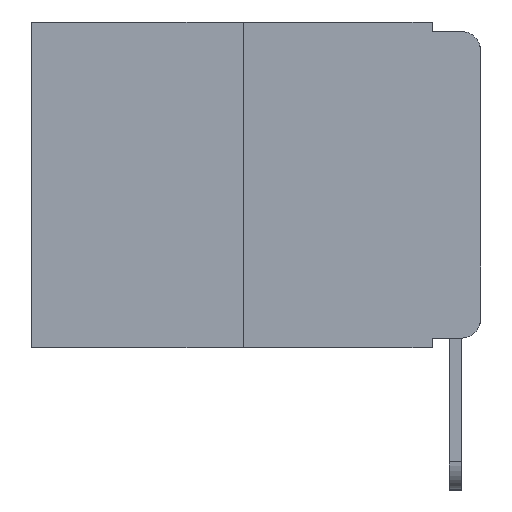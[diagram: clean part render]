
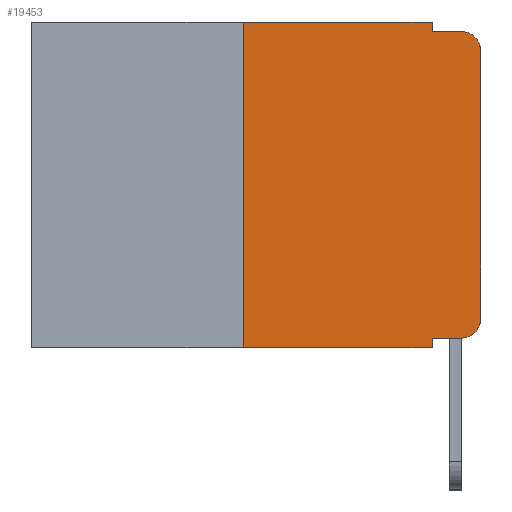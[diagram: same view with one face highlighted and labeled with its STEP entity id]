
A CAD part, left-side view. The second image highlights one B-rep face of the part: STEP entity #19453.
In plain terms, the highlighted planar face has unit normal (-1, 0, 0).
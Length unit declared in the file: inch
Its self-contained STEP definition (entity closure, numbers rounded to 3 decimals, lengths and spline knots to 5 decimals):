
#561 = CARTESIAN_POINT ( 'NONE',  ( 0., 0.02, -0.333 ) ) ;
#791 = LINE ( 'NONE', #21760, #6153 ) ;
#877 = CARTESIAN_POINT ( 'NONE',  ( 0., 0.473, 0. ) ) ;
#1076 = EDGE_CURVE ( 'NONE', #20638, #2877, #19353, .T. ) ;
#1292 = VERTEX_POINT ( 'NONE', #16886 ) ;
#1358 = LINE ( 'NONE', #10481, #18999 ) ;
#1456 = ORIENTED_EDGE ( 'NONE', *, *, #20039, .T. ) ;
#1734 = ORIENTED_EDGE ( 'NONE', *, *, #22478, .F. ) ;
#2273 = VERTEX_POINT ( 'NONE', #11012 ) ;
#2295 = ORIENTED_EDGE ( 'NONE', *, *, #1076, .T. ) ;
#2457 = CARTESIAN_POINT ( 'NONE',  ( 0., 0.051, -0.343 ) ) ;
#2680 = EDGE_CURVE ( 'NONE', #2273, #12770, #791, .T. ) ;
#2717 = EDGE_CURVE ( 'NONE', #8320, #11078, #9775, .T. ) ;
#2746 = VECTOR ( 'NONE', #3614, 39.37008 ) ;
#2760 = VECTOR ( 'NONE', #19916, 39.37008 ) ;
#2839 = ORIENTED_EDGE ( 'NONE', *, *, #9731, .F. ) ;
#2877 = VERTEX_POINT ( 'NONE', #6705 ) ;
#3085 = CIRCLE ( 'NONE', #3307, 0.02 ) ;
#3307 = AXIS2_PLACEMENT_3D ( 'NONE', #3988, #16331, #5822 ) ;
#3327 = LINE ( 'NONE', #18181, #2760 ) ;
#3405 = VERTEX_POINT ( 'NONE', #18435 ) ;
#3503 = DIRECTION ( 'NONE',  ( 0., -1., 0. ) ) ;
#3614 = DIRECTION ( 'NONE',  ( 0., 0., 1. ) ) ;
#3872 = VERTEX_POINT ( 'NONE', #16247 ) ;
#3988 = CARTESIAN_POINT ( 'NONE',  ( 0., 0.02, -0.03 ) ) ;
#4575 = VECTOR ( 'NONE', #14661, 39.37008 ) ;
#5822 = DIRECTION ( 'NONE',  ( 0., 0., -1. ) ) ;
#6153 = VECTOR ( 'NONE', #13206, 39.37008 ) ;
#6234 = ORIENTED_EDGE ( 'NONE', *, *, #8613, .T. ) ;
#6241 = DIRECTION ( 'NONE',  ( 0., -1., 0. ) ) ;
#6357 = PLANE ( 'NONE',  #7781 ) ;
#6705 = CARTESIAN_POINT ( 'NONE',  ( 0., 0., -0.313 ) ) ;
#7355 = ORIENTED_EDGE ( 'NONE', *, *, #2717, .F. ) ;
#7563 = LINE ( 'NONE', #8974, #2746 ) ;
#7781 = AXIS2_PLACEMENT_3D ( 'NONE', #18409, #22014, #11719 ) ;
#8052 = DIRECTION ( 'NONE',  ( 0., -1., 0. ) ) ;
#8320 = VERTEX_POINT ( 'NONE', #20293 ) ;
#8613 = EDGE_CURVE ( 'NONE', #20926, #11078, #3085, .T. ) ;
#8681 = VECTOR ( 'NONE', #8052, 39.37008 ) ;
#8935 = AXIS2_PLACEMENT_3D ( 'NONE', #9504, #21610, #11295 ) ;
#8974 = CARTESIAN_POINT ( 'NONE',  ( 0., 0.25, 0. ) ) ;
#9058 = ORIENTED_EDGE ( 'NONE', *, *, #14055, .T. ) ;
#9296 = ORIENTED_EDGE ( 'NONE', *, *, #10811, .T. ) ;
#9455 = CARTESIAN_POINT ( 'NONE',  ( 0., 0.02, -0.01 ) ) ;
#9504 = CARTESIAN_POINT ( 'NONE',  ( 0., 0.02, -0.313 ) ) ;
#9731 = EDGE_CURVE ( 'NONE', #3405, #3872, #7563, .T. ) ;
#9775 = LINE ( 'NONE', #18458, #8681 ) ;
#10481 = CARTESIAN_POINT ( 'NONE',  ( 0., 0., 0. ) ) ;
#10811 = EDGE_CURVE ( 'NONE', #2877, #20926, #1358, .T. ) ;
#10892 = LINE ( 'NONE', #877, #20084 ) ;
#11012 = CARTESIAN_POINT ( 'NONE',  ( 0., 0.051, -0.333 ) ) ;
#11078 = VERTEX_POINT ( 'NONE', #9455 ) ;
#11295 = DIRECTION ( 'NONE',  ( 0., 0., -1. ) ) ;
#11719 = DIRECTION ( 'NONE',  ( 0., 0., -1. ) ) ;
#12176 = DIRECTION ( 'NONE',  ( 0., 0., 1. ) ) ;
#12417 = CARTESIAN_POINT ( 'NONE',  ( 0., 0.051, -0.333 ) ) ;
#12770 = VERTEX_POINT ( 'NONE', #2457 ) ;
#13206 = DIRECTION ( 'NONE',  ( 0., 0., -1. ) ) ;
#13997 = VECTOR ( 'NONE', #3503, 39.37008 ) ;
#14022 = LINE ( 'NONE', #18099, #4575 ) ;
#14055 = EDGE_CURVE ( 'NONE', #2273, #20638, #22558, .T. ) ;
#14277 = EDGE_CURVE ( 'NONE', #1292, #8320, #14022, .T. ) ;
#14661 = DIRECTION ( 'NONE',  ( 0., 0., -1. ) ) ;
#15991 = EDGE_LOOP ( 'NONE', ( #9296, #6234, #7355, #18263, #1734, #2839, #1456, #16687, #9058, #2295 ) ) ;
#16247 = CARTESIAN_POINT ( 'NONE',  ( 0., 0.25, 0. ) ) ;
#16331 = DIRECTION ( 'NONE',  ( -1., 0., 0. ) ) ;
#16687 = ORIENTED_EDGE ( 'NONE', *, *, #2680, .F. ) ;
#16886 = CARTESIAN_POINT ( 'NONE',  ( 0., 0.051, 0. ) ) ;
#18099 = CARTESIAN_POINT ( 'NONE',  ( 0., 0.051, 0. ) ) ;
#18181 = CARTESIAN_POINT ( 'NONE',  ( 0., 0.473, -0.343 ) ) ;
#18263 = ORIENTED_EDGE ( 'NONE', *, *, #14277, .F. ) ;
#18409 = CARTESIAN_POINT ( 'NONE',  ( 0., 0.473, 0. ) ) ;
#18435 = CARTESIAN_POINT ( 'NONE',  ( 0., 0.25, -0.343 ) ) ;
#18458 = CARTESIAN_POINT ( 'NONE',  ( 0., 0.051, -0.01 ) ) ;
#18999 = VECTOR ( 'NONE', #12176, 39.37008 ) ;
#19353 = CIRCLE ( 'NONE', #8935, 0.02 ) ;
#19453 = ADVANCED_FACE ( 'NONE', ( #20672 ), #6357, .F. ) ;
#19916 = DIRECTION ( 'NONE',  ( 0., -1., 0. ) ) ;
#20039 = EDGE_CURVE ( 'NONE', #3405, #12770, #3327, .T. ) ;
#20084 = VECTOR ( 'NONE', #6241, 39.37008 ) ;
#20293 = CARTESIAN_POINT ( 'NONE',  ( 0., 0.051, -0.01 ) ) ;
#20638 = VERTEX_POINT ( 'NONE', #561 ) ;
#20672 = FACE_OUTER_BOUND ( 'NONE', #15991, .T. ) ;
#20926 = VERTEX_POINT ( 'NONE', #22425 ) ;
#21610 = DIRECTION ( 'NONE',  ( -1., 0., 0. ) ) ;
#21760 = CARTESIAN_POINT ( 'NONE',  ( 0., 0.051, 0. ) ) ;
#22014 = DIRECTION ( 'NONE',  ( 1., 0., 0. ) ) ;
#22425 = CARTESIAN_POINT ( 'NONE',  ( 0., 0., -0.03 ) ) ;
#22478 = EDGE_CURVE ( 'NONE', #3872, #1292, #10892, .T. ) ;
#22558 = LINE ( 'NONE', #12417, #13997 ) ;
